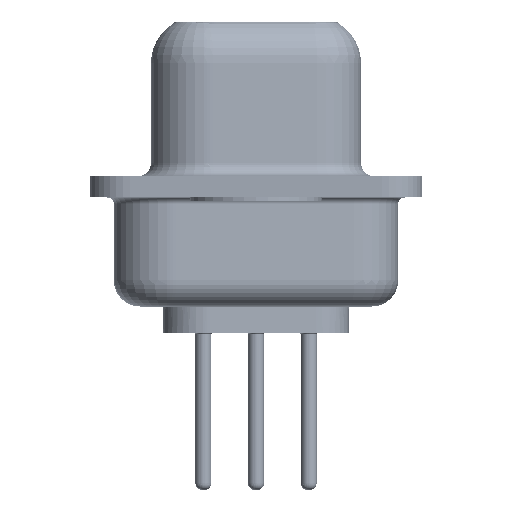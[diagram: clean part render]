
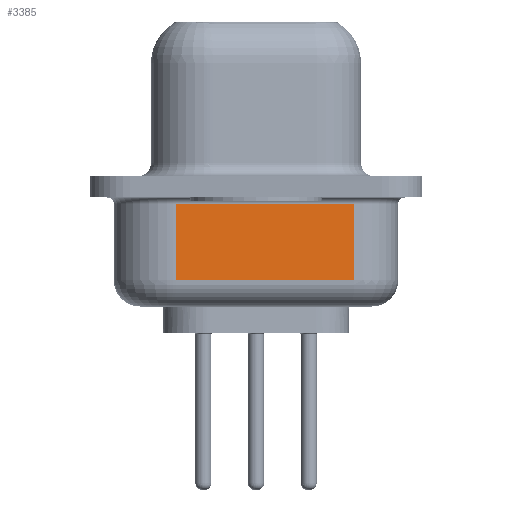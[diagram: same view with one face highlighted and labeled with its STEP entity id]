
A CAD part, left-side view. The second image highlights one B-rep face of the part: STEP entity #3385.
In plain terms, the highlighted planar face has unit normal (-0.985, -0.174, 0).
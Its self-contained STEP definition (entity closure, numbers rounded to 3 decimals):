
#2438 = VECTOR ( 'NONE', #31727, 1000. ) ;
#3070 = VECTOR ( 'NONE', #32676, 1000. ) ;
#3291 = CARTESIAN_POINT ( 'NONE',  ( 2.88, 3.003, -4.5 ) ) ;
#3385 = ADVANCED_FACE ( 'NONE', ( #17080 ), #28161, .F. ) ;
#3463 = CARTESIAN_POINT ( 'NONE',  ( 4.062, -3.697, -0.65 ) ) ;
#3642 = LINE ( 'NONE', #23011, #18465 ) ;
#5608 = EDGE_CURVE ( 'NONE', #34362, #32440, #17708, .T. ) ;
#6346 = CARTESIAN_POINT ( 'NONE',  ( 2.88, 3.003, -3.5 ) ) ;
#6561 = ORIENTED_EDGE ( 'NONE', *, *, #15021, .T. ) ;
#6937 = EDGE_CURVE ( 'NONE', #34362, #35159, #15035, .T. ) ;
#7918 = CARTESIAN_POINT ( 'NONE',  ( 2.88, 3.003, -0.65 ) ) ;
#10690 = LINE ( 'NONE', #19375, #3070 ) ;
#13095 = VERTEX_POINT ( 'NONE', #3463 ) ;
#14138 = CARTESIAN_POINT ( 'NONE',  ( 4.062, -3.697, -3.5 ) ) ;
#14359 = ORIENTED_EDGE ( 'NONE', *, *, #5608, .F. ) ;
#15021 = EDGE_CURVE ( 'NONE', #13095, #32440, #10690, .T. ) ;
#15035 = LINE ( 'NONE', #6346, #20803 ) ;
#17080 = FACE_OUTER_BOUND ( 'NONE', #34897, .T. ) ;
#17258 = DIRECTION ( 'NONE',  ( 0.985, 0.174, 0. ) ) ;
#17708 = LINE ( 'NONE', #20972, #2438 ) ;
#18465 = VECTOR ( 'NONE', #23382, 1000. ) ;
#19375 = CARTESIAN_POINT ( 'NONE',  ( 2.88, 3.003, -0.65 ) ) ;
#20201 = EDGE_CURVE ( 'NONE', #35159, #13095, #3642, .T. ) ;
#20803 = VECTOR ( 'NONE', #35201, 1000. ) ;
#20972 = CARTESIAN_POINT ( 'NONE',  ( 2.88, 3.003, -4.5 ) ) ;
#21205 = ORIENTED_EDGE ( 'NONE', *, *, #20201, .T. ) ;
#23011 = CARTESIAN_POINT ( 'NONE',  ( 4.062, -3.697, -4.5 ) ) ;
#23382 = DIRECTION ( 'NONE',  ( 0., 0., 1. ) ) ;
#26110 = ORIENTED_EDGE ( 'NONE', *, *, #6937, .T. ) ;
#28161 = PLANE ( 'NONE',  #30979 ) ;
#28337 = DIRECTION ( 'NONE',  ( -0.174, 0.985, 0. ) ) ;
#30979 = AXIS2_PLACEMENT_3D ( 'NONE', #3291, #17258, #28337 ) ;
#31727 = DIRECTION ( 'NONE',  ( 0., 0., 1. ) ) ;
#32440 = VERTEX_POINT ( 'NONE', #7918 ) ;
#32676 = DIRECTION ( 'NONE',  ( -0.174, 0.985, 0. ) ) ;
#34050 = CARTESIAN_POINT ( 'NONE',  ( 2.88, 3.003, -3.5 ) ) ;
#34362 = VERTEX_POINT ( 'NONE', #34050 ) ;
#34897 = EDGE_LOOP ( 'NONE', ( #14359, #26110, #21205, #6561 ) ) ;
#35159 = VERTEX_POINT ( 'NONE', #14138 ) ;
#35201 = DIRECTION ( 'NONE',  ( 0.174, -0.985, 0. ) ) ;
